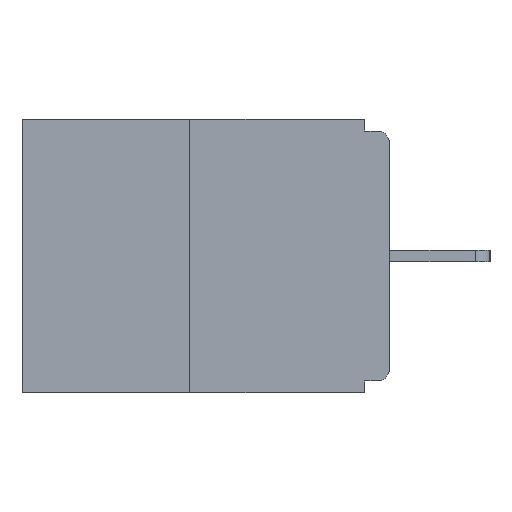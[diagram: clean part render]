
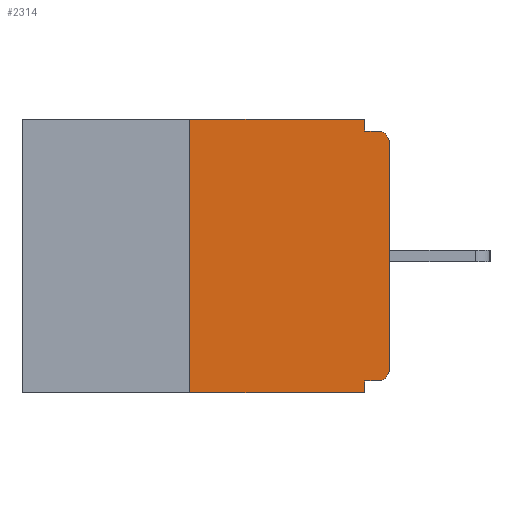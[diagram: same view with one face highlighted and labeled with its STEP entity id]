
A CAD part, left-side view. The second image highlights one B-rep face of the part: STEP entity #2314.
In plain terms, the highlighted planar face has unit normal (-1, 0, 0).
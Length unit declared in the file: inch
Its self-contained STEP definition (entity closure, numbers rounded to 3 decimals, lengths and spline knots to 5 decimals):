
#9 = DIRECTION ( 'NONE',  ( 0., 0., -1. ) ) ;
#43 = DIRECTION ( 'NONE',  ( 0., 0., -1. ) ) ;
#181 = VERTEX_POINT ( 'NONE', #3431 ) ;
#680 = EDGE_CURVE ( 'NONE', #19324, #4792, #8279, .T. ) ;
#774 = CARTESIAN_POINT ( 'NONE',  ( 0., 0., -0.328 ) ) ;
#1010 = CARTESIAN_POINT ( 'NONE',  ( 0., 0.031, -0.328 ) ) ;
#1098 = DIRECTION ( 'NONE',  ( -1., 0., 0. ) ) ;
#1215 = AXIS2_PLACEMENT_3D ( 'NONE', #10881, #24425, #12836 ) ;
#1705 = ORIENTED_EDGE ( 'NONE', *, *, #17209, .T. ) ;
#1816 = CARTESIAN_POINT ( 'NONE',  ( 0., 0., -0.015 ) ) ;
#2314 = ADVANCED_FACE ( 'NONE', ( #11896 ), #19382, .F. ) ;
#2757 = CARTESIAN_POINT ( 'NONE',  ( 0., 0.031, 0. ) ) ;
#3234 = DIRECTION ( 'NONE',  ( 0., 0., -1. ) ) ;
#3263 = DIRECTION ( 'NONE',  ( 1., 0., 0. ) ) ;
#3431 = CARTESIAN_POINT ( 'NONE',  ( 0., 0.25, 0. ) ) ;
#3559 = EDGE_CURVE ( 'NONE', #4792, #21851, #9415, .T. ) ;
#3831 = VECTOR ( 'NONE', #17911, 39.37008 ) ;
#4079 = LINE ( 'NONE', #17648, #19168 ) ;
#4541 = DIRECTION ( 'NONE',  ( 0., 0., 1. ) ) ;
#4673 = EDGE_LOOP ( 'NONE', ( #23650, #14220, #1705, #13636, #17430, #24098, #9827, #20498, #8444, #6628 ) ) ;
#4716 = VECTOR ( 'NONE', #11987, 39.37008 ) ;
#4792 = VERTEX_POINT ( 'NONE', #20411 ) ;
#5213 = LINE ( 'NONE', #21772, #20248 ) ;
#5410 = VECTOR ( 'NONE', #4541, 39.37008 ) ;
#5425 = CIRCLE ( 'NONE', #1215, 0.015 ) ;
#5478 = AXIS2_PLACEMENT_3D ( 'NONE', #20243, #3263, #3234 ) ;
#5659 = EDGE_CURVE ( 'NONE', #181, #9192, #4079, .T. ) ;
#5678 = CARTESIAN_POINT ( 'NONE',  ( 0., 0.015, -0.313 ) ) ;
#5735 = DIRECTION ( 'NONE',  ( 0., 0., -1. ) ) ;
#6628 = ORIENTED_EDGE ( 'NONE', *, *, #16609, .F. ) ;
#7144 = EDGE_CURVE ( 'NONE', #21904, #19043, #13339, .T. ) ;
#8175 = CARTESIAN_POINT ( 'NONE',  ( 0., 0.031, 0. ) ) ;
#8279 = CIRCLE ( 'NONE', #9156, 0.015 ) ;
#8444 = ORIENTED_EDGE ( 'NONE', *, *, #7144, .F. ) ;
#9156 = AXIS2_PLACEMENT_3D ( 'NONE', #5678, #1098, #5735 ) ;
#9192 = VERTEX_POINT ( 'NONE', #2757 ) ;
#9415 = LINE ( 'NONE', #10011, #4716 ) ;
#9827 = ORIENTED_EDGE ( 'NONE', *, *, #3559, .T. ) ;
#10011 = CARTESIAN_POINT ( 'NONE',  ( 0., 0., 0. ) ) ;
#10478 = EDGE_CURVE ( 'NONE', #21851, #19043, #5425, .T. ) ;
#10726 = LINE ( 'NONE', #16377, #5410 ) ;
#10881 = CARTESIAN_POINT ( 'NONE',  ( 0., 0.015, -0.03 ) ) ;
#11571 = CARTESIAN_POINT ( 'NONE',  ( 0., 0.015, -0.328 ) ) ;
#11896 = FACE_OUTER_BOUND ( 'NONE', #4673, .T. ) ;
#11987 = DIRECTION ( 'NONE',  ( 0., 0., 1. ) ) ;
#12103 = VECTOR ( 'NONE', #19934, 39.37008 ) ;
#12836 = DIRECTION ( 'NONE',  ( 0., 0., -1. ) ) ;
#13099 = VERTEX_POINT ( 'NONE', #1010 ) ;
#13339 = LINE ( 'NONE', #1816, #12103 ) ;
#13636 = ORIENTED_EDGE ( 'NONE', *, *, #20793, .F. ) ;
#14220 = ORIENTED_EDGE ( 'NONE', *, *, #22650, .F. ) ;
#14319 = EDGE_CURVE ( 'NONE', #19324, #13099, #23004, .T. ) ;
#14653 = CARTESIAN_POINT ( 'NONE',  ( 0., 0.015, -0.015 ) ) ;
#14734 = DIRECTION ( 'NONE',  ( 0., 1., 0. ) ) ;
#16032 = VERTEX_POINT ( 'NONE', #23416 ) ;
#16377 = CARTESIAN_POINT ( 'NONE',  ( 0., 0.25, 0. ) ) ;
#16609 = EDGE_CURVE ( 'NONE', #9192, #21904, #19259, .T. ) ;
#17209 = EDGE_CURVE ( 'NONE', #16032, #20598, #24646, .T. ) ;
#17430 = ORIENTED_EDGE ( 'NONE', *, *, #14319, .F. ) ;
#17618 = CARTESIAN_POINT ( 'NONE',  ( 0., 0., -0.03 ) ) ;
#17648 = CARTESIAN_POINT ( 'NONE',  ( 0., 0.46, 0. ) ) ;
#17859 = CARTESIAN_POINT ( 'NONE',  ( 0., 0.031, -0.015 ) ) ;
#17898 = VECTOR ( 'NONE', #14734, 39.37008 ) ;
#17911 = DIRECTION ( 'NONE',  ( 0., -1., 0. ) ) ;
#19043 = VERTEX_POINT ( 'NONE', #14653 ) ;
#19168 = VECTOR ( 'NONE', #19779, 39.37008 ) ;
#19259 = LINE ( 'NONE', #8175, #23784 ) ;
#19324 = VERTEX_POINT ( 'NONE', #11571 ) ;
#19382 = PLANE ( 'NONE',  #5478 ) ;
#19779 = DIRECTION ( 'NONE',  ( 0., -1., 0. ) ) ;
#19934 = DIRECTION ( 'NONE',  ( 0., -1., 0. ) ) ;
#20243 = CARTESIAN_POINT ( 'NONE',  ( 0., 0.46, 0. ) ) ;
#20248 = VECTOR ( 'NONE', #9, 39.37008 ) ;
#20411 = CARTESIAN_POINT ( 'NONE',  ( 0., 0., -0.313 ) ) ;
#20498 = ORIENTED_EDGE ( 'NONE', *, *, #10478, .T. ) ;
#20598 = VERTEX_POINT ( 'NONE', #24964 ) ;
#20793 = EDGE_CURVE ( 'NONE', #13099, #20598, #5213, .T. ) ;
#21684 = CARTESIAN_POINT ( 'NONE',  ( 0., 0.46, -0.343 ) ) ;
#21772 = CARTESIAN_POINT ( 'NONE',  ( 0., 0.031, -0.343 ) ) ;
#21851 = VERTEX_POINT ( 'NONE', #17618 ) ;
#21904 = VERTEX_POINT ( 'NONE', #17859 ) ;
#22650 = EDGE_CURVE ( 'NONE', #16032, #181, #10726, .T. ) ;
#23004 = LINE ( 'NONE', #774, #17898 ) ;
#23416 = CARTESIAN_POINT ( 'NONE',  ( 0., 0.25, -0.343 ) ) ;
#23650 = ORIENTED_EDGE ( 'NONE', *, *, #5659, .F. ) ;
#23784 = VECTOR ( 'NONE', #43, 39.37008 ) ;
#24098 = ORIENTED_EDGE ( 'NONE', *, *, #680, .T. ) ;
#24425 = DIRECTION ( 'NONE',  ( -1., 0., 0. ) ) ;
#24646 = LINE ( 'NONE', #21684, #3831 ) ;
#24964 = CARTESIAN_POINT ( 'NONE',  ( 0., 0.031, -0.343 ) ) ;
